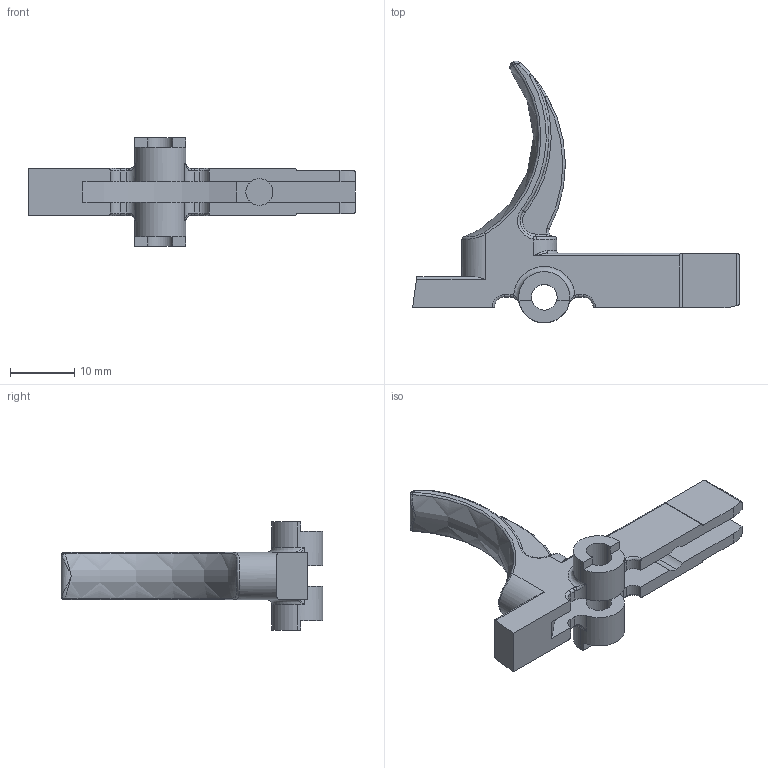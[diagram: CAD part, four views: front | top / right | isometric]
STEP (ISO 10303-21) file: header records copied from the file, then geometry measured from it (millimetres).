
FILE_DESCRIPTION((''),'2;1');
FILE_NAME('AUTO_TRIGGER','2019-01-20T17:52:54',('Cust'),(''),'CREO PARAMETRIC BY PTC INC, 2018300','CREO PARAMETRIC BY PTC INC, 2018300','');
FILE_SCHEMA(('AUTOMOTIVE_DESIGN { 1 0 10303 214 1 1 1 1 }'));
Length unit declared in the file: inch
Products named in the file (1): AUTO_TRIGGER
Bounding box: 51.01 x 40.83 x 16.87 mm (x, y, z)
Volume: 3332.9 mm3; surface area: 3176.8 mm2
Topology: 1 solids, 1 shells, 148 faces, 420 edges, 258 vertices
Faces by surface type: cylinder 51, plane 39, torus 32, bspline 23, sphere 2, revolution 1
Entity records: 6906 total; most frequent: CARTESIAN_POINT 1895, ORIENTED_EDGE 812, DIRECTION 781, PRESENTATION_STYLE_ASSIGNMENT 409, STYLED_ITEM 407, CURVE_STYLE 406, EDGE_CURVE 406, AXIS2_PLACEMENT_3D 319
